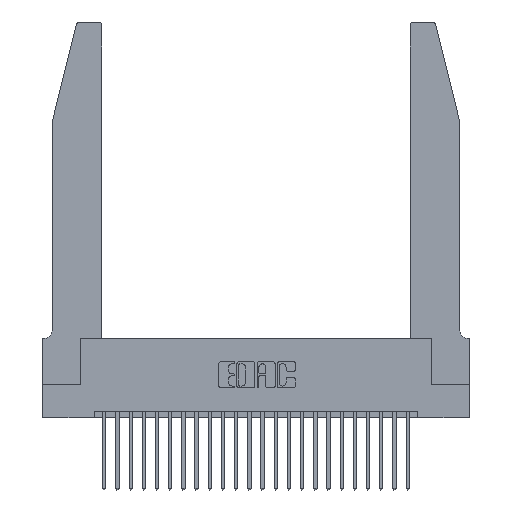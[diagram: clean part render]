
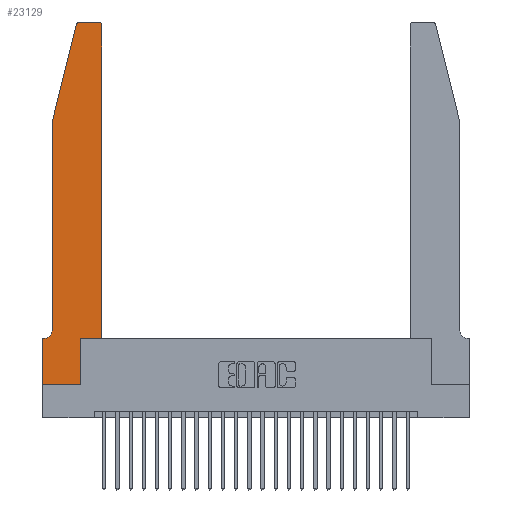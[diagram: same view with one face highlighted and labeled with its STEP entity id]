
A CAD part, top view. The second image highlights one B-rep face of the part: STEP entity #23129.
In plain terms, the highlighted planar face has unit normal (0, 0, 1).
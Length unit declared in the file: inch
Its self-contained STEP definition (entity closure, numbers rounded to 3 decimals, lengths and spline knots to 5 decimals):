
#288 = DIRECTION ( 'NONE',  ( 1., 0., 0. ) ) ;
#311 = CARTESIAN_POINT ( 'NONE',  ( 0.0755, 0.35, 0.37 ) ) ;
#339 = LINE ( 'NONE', #311, #11253 ) ;
#1462 = CARTESIAN_POINT ( 'NONE',  ( 0.284, 2.72, 0.37 ) ) ;
#1519 = CARTESIAN_POINT ( 'NONE',  ( 0.2865, 0.35, 0.37 ) ) ;
#1779 = LINE ( 'NONE', #8537, #3048 ) ;
#2056 = CARTESIAN_POINT ( 'NONE',  ( 0.25487, 2.72718, 0.37 ) ) ;
#2261 = VECTOR ( 'NONE', #13192, 39.37008 ) ;
#2651 = CARTESIAN_POINT ( 'NONE',  ( 0.4505, 0.35, 0.37 ) ) ;
#2679 = VERTEX_POINT ( 'NONE', #2056 ) ;
#2699 = VECTOR ( 'NONE', #18286, 39.37008 ) ;
#2903 = LINE ( 'NONE', #7038, #2261 ) ;
#3048 = VECTOR ( 'NONE', #18631, 39.37008 ) ;
#3496 = DIRECTION ( 'NONE',  ( 1., 0., 0. ) ) ;
#3745 = VERTEX_POINT ( 'NONE', #22088 ) ;
#4111 = ORIENTED_EDGE ( 'NONE', *, *, #6140, .T. ) ;
#4127 = EDGE_CURVE ( 'NONE', #22894, #21743, #2903, .T. ) ;
#4256 = AXIS2_PLACEMENT_3D ( 'NONE', #20720, #8757, #22678 ) ;
#4666 = ORIENTED_EDGE ( 'NONE', *, *, #24041, .T. ) ;
#4845 = ORIENTED_EDGE ( 'NONE', *, *, #23215, .T. ) ;
#5210 = CARTESIAN_POINT ( 'NONE',  ( 0.4205, 2.75, 0.37 ) ) ;
#5415 = ORIENTED_EDGE ( 'NONE', *, *, #19229, .T. ) ;
#6140 = EDGE_CURVE ( 'NONE', #22670, #23782, #18379, .T. ) ;
#6252 = CARTESIAN_POINT ( 'NONE',  ( 0.0755, 2., 0.37 ) ) ;
#6570 = ORIENTED_EDGE ( 'NONE', *, *, #14375, .T. ) ;
#7038 = CARTESIAN_POINT ( 'NONE',  ( 0.0755, 2., 0.37 ) ) ;
#7056 = LINE ( 'NONE', #7743, #17190 ) ;
#7195 = CIRCLE ( 'NONE', #22935, 0.03 ) ;
#7332 = CARTESIAN_POINT ( 'NONE',  ( 0., 0.35, 0.37 ) ) ;
#7743 = CARTESIAN_POINT ( 'NONE',  ( 0., 0., 0.37 ) ) ;
#8329 = VECTOR ( 'NONE', #20920, 39.37008 ) ;
#8389 = ORIENTED_EDGE ( 'NONE', *, *, #24687, .T. ) ;
#8537 = CARTESIAN_POINT ( 'NONE',  ( 0.0755, 2., 0.37 ) ) ;
#8757 = DIRECTION ( 'NONE',  ( 0., 0., 1. ) ) ;
#9323 = VERTEX_POINT ( 'NONE', #18831 ) ;
#9539 = EDGE_CURVE ( 'NONE', #23782, #25802, #18193, .T. ) ;
#9679 = CIRCLE ( 'NONE', #17570, 0.07 ) ;
#9756 = DIRECTION ( 'NONE',  ( 1., 0., 0. ) ) ;
#9885 = ORIENTED_EDGE ( 'NONE', *, *, #16817, .T. ) ;
#10277 = VERTEX_POINT ( 'NONE', #24009 ) ;
#10279 = DIRECTION ( 'NONE',  ( 0., 0., -1. ) ) ;
#10993 = DIRECTION ( 'NONE',  ( -1., 0., 0. ) ) ;
#11253 = VECTOR ( 'NONE', #14600, 39.37008 ) ;
#11854 = VERTEX_POINT ( 'NONE', #17301 ) ;
#12891 = VECTOR ( 'NONE', #10993, 39.37008 ) ;
#13192 = DIRECTION ( 'NONE',  ( 0., -1., 0. ) ) ;
#13864 = FACE_OUTER_BOUND ( 'NONE', #25446, .T. ) ;
#14375 = EDGE_CURVE ( 'NONE', #9323, #10277, #17973, .T. ) ;
#14572 = EDGE_CURVE ( 'NONE', #18514, #16396, #18891, .T. ) ;
#14600 = DIRECTION ( 'NONE',  ( -1., 0., 0. ) ) ;
#14730 = CARTESIAN_POINT ( 'NONE',  ( 0.0755, 0.42, 0.37 ) ) ;
#14749 = ORIENTED_EDGE ( 'NONE', *, *, #9539, .T. ) ;
#15712 = DIRECTION ( 'NONE',  ( 0., 0., 1. ) ) ;
#15763 = LINE ( 'NONE', #16603, #25597 ) ;
#16295 = CARTESIAN_POINT ( 'NONE',  ( 0.2865, 0.35, 0.37 ) ) ;
#16394 = EDGE_CURVE ( 'NONE', #10277, #18514, #7056, .T. ) ;
#16396 = VERTEX_POINT ( 'NONE', #1519 ) ;
#16603 = CARTESIAN_POINT ( 'NONE',  ( 0.4505, 0.35, 0.37 ) ) ;
#16817 = EDGE_CURVE ( 'NONE', #11854, #22670, #20215, .T. ) ;
#17190 = VECTOR ( 'NONE', #9756, 39.37008 ) ;
#17301 = CARTESIAN_POINT ( 'NONE',  ( 0.4505, 0.35, 0.37 ) ) ;
#17570 = AXIS2_PLACEMENT_3D ( 'NONE', #22207, #10279, #24169 ) ;
#17705 = DIRECTION ( 'NONE',  ( 0., -1., 0. ) ) ;
#17973 = LINE ( 'NONE', #23493, #22543 ) ;
#18193 = LINE ( 'NONE', #24850, #12891 ) ;
#18286 = DIRECTION ( 'NONE',  ( 0., 1., 0. ) ) ;
#18379 = CIRCLE ( 'NONE', #4256, 0.03 ) ;
#18459 = EDGE_CURVE ( 'NONE', #2679, #22894, #1779, .T. ) ;
#18461 = ORIENTED_EDGE ( 'NONE', *, *, #4127, .T. ) ;
#18514 = VERTEX_POINT ( 'NONE', #22634 ) ;
#18564 = ORIENTED_EDGE ( 'NONE', *, *, #18459, .T. ) ;
#18631 = DIRECTION ( 'NONE',  ( -0.239, -0.971, 0. ) ) ;
#18831 = CARTESIAN_POINT ( 'NONE',  ( 0., 0.35, 0.37 ) ) ;
#18891 = LINE ( 'NONE', #16295, #2699 ) ;
#19020 = AXIS2_PLACEMENT_3D ( 'NONE', #7332, #21150, #23269 ) ;
#19229 = EDGE_CURVE ( 'NONE', #16396, #11854, #15763, .T. ) ;
#19359 = PLANE ( 'NONE',  #19020 ) ;
#20215 = LINE ( 'NONE', #2651, #8329 ) ;
#20476 = ORIENTED_EDGE ( 'NONE', *, *, #14572, .T. ) ;
#20720 = CARTESIAN_POINT ( 'NONE',  ( 0.4205, 2.72, 0.37 ) ) ;
#20920 = DIRECTION ( 'NONE',  ( 0., 1., 0. ) ) ;
#21150 = DIRECTION ( 'NONE',  ( 0., 0., 1. ) ) ;
#21743 = VERTEX_POINT ( 'NONE', #14730 ) ;
#22088 = CARTESIAN_POINT ( 'NONE',  ( 0.0055, 0.35, 0.37 ) ) ;
#22207 = CARTESIAN_POINT ( 'NONE',  ( 0.0055, 0.42, 0.37 ) ) ;
#22543 = VECTOR ( 'NONE', #17705, 39.37008 ) ;
#22634 = CARTESIAN_POINT ( 'NONE',  ( 0.2865, 0., 0.37 ) ) ;
#22670 = VERTEX_POINT ( 'NONE', #25534 ) ;
#22678 = DIRECTION ( 'NONE',  ( 1., 0., 0. ) ) ;
#22894 = VERTEX_POINT ( 'NONE', #6252 ) ;
#22935 = AXIS2_PLACEMENT_3D ( 'NONE', #1462, #15712, #3496 ) ;
#23129 = ADVANCED_FACE ( 'NONE', ( #13864 ), #19359, .T. ) ;
#23215 = EDGE_CURVE ( 'NONE', #25802, #2679, #7195, .T. ) ;
#23269 = DIRECTION ( 'NONE',  ( 1., 0., 0. ) ) ;
#23493 = CARTESIAN_POINT ( 'NONE',  ( 0., 0., 0.37 ) ) ;
#23782 = VERTEX_POINT ( 'NONE', #5210 ) ;
#24009 = CARTESIAN_POINT ( 'NONE',  ( 0., 0., 0.37 ) ) ;
#24041 = EDGE_CURVE ( 'NONE', #21743, #3745, #9679, .T. ) ;
#24104 = CARTESIAN_POINT ( 'NONE',  ( 0.284, 2.75, 0.37 ) ) ;
#24169 = DIRECTION ( 'NONE',  ( -1., 0., 0. ) ) ;
#24426 = ORIENTED_EDGE ( 'NONE', *, *, #16394, .T. ) ;
#24687 = EDGE_CURVE ( 'NONE', #3745, #9323, #339, .T. ) ;
#24850 = CARTESIAN_POINT ( 'NONE',  ( 0.2605, 2.75, 0.37 ) ) ;
#25446 = EDGE_LOOP ( 'NONE', ( #14749, #4845, #18564, #18461, #4666, #8389, #6570, #24426, #20476, #5415, #9885, #4111 ) ) ;
#25534 = CARTESIAN_POINT ( 'NONE',  ( 0.4505, 2.72, 0.37 ) ) ;
#25597 = VECTOR ( 'NONE', #288, 39.37008 ) ;
#25802 = VERTEX_POINT ( 'NONE', #24104 ) ;
